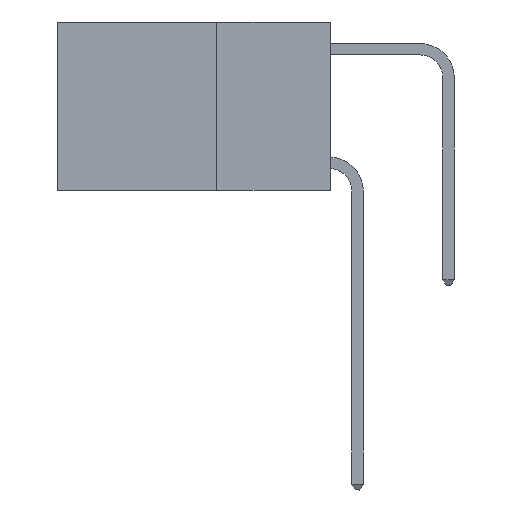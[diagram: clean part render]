
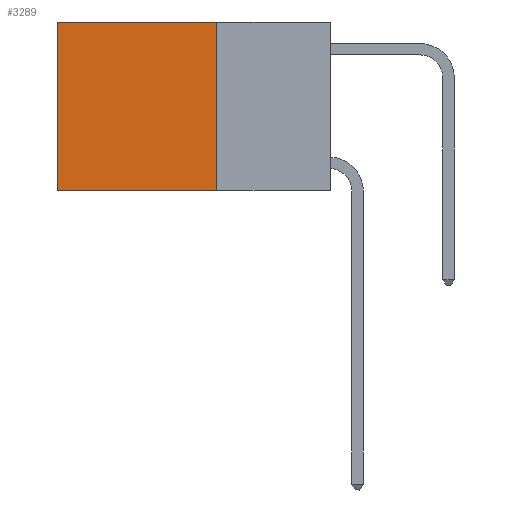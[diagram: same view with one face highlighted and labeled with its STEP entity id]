
A CAD part, left-side view. The second image highlights one B-rep face of the part: STEP entity #3289.
In plain terms, the highlighted planar face has unit normal (-1, 0, 0).
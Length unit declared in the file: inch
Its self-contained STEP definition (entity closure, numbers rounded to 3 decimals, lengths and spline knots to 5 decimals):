
#156 = PLANE ( 'NONE',  #4739 ) ;
#250 = LINE ( 'NONE', #12673, #16236 ) ;
#1476 = EDGE_LOOP ( 'NONE', ( #14057, #16489, #4400, #17234 ) ) ;
#1740 = DIRECTION ( 'NONE',  ( 0., 0., -1. ) ) ;
#2521 = VERTEX_POINT ( 'NONE', #5800 ) ;
#3289 = ADVANCED_FACE ( 'NONE', ( #7120 ), #156, .F. ) ;
#4400 = ORIENTED_EDGE ( 'NONE', *, *, #5109, .F. ) ;
#4739 = AXIS2_PLACEMENT_3D ( 'NONE', #4765, #10937, #1740 ) ;
#4765 = CARTESIAN_POINT ( 'NONE',  ( 0.2625, 0.25, 0. ) ) ;
#4880 = VECTOR ( 'NONE', #14399, 39.37008 ) ;
#5109 = EDGE_CURVE ( 'NONE', #18228, #11532, #250, .T. ) ;
#5800 = CARTESIAN_POINT ( 'NONE',  ( 0.2625, 0.6, 0. ) ) ;
#7120 = FACE_OUTER_BOUND ( 'NONE', #1476, .T. ) ;
#8067 = VECTOR ( 'NONE', #8450, 39.37008 ) ;
#8450 = DIRECTION ( 'NONE',  ( 0., 0., -1. ) ) ;
#8711 = EDGE_CURVE ( 'NONE', #18228, #2521, #14428, .T. ) ;
#9574 = CARTESIAN_POINT ( 'NONE',  ( 0.2625, 0.25, -0.37 ) ) ;
#10260 = VECTOR ( 'NONE', #14422, 39.37008 ) ;
#10937 = DIRECTION ( 'NONE',  ( 1., 0., 0. ) ) ;
#11504 = VERTEX_POINT ( 'NONE', #14237 ) ;
#11532 = VERTEX_POINT ( 'NONE', #9574 ) ;
#12673 = CARTESIAN_POINT ( 'NONE',  ( 0.2625, 0.25, 0. ) ) ;
#12789 = CARTESIAN_POINT ( 'NONE',  ( 0.2625, 0.25, -0.37 ) ) ;
#14057 = ORIENTED_EDGE ( 'NONE', *, *, #14212, .T. ) ;
#14212 = EDGE_CURVE ( 'NONE', #2521, #11504, #16334, .T. ) ;
#14237 = CARTESIAN_POINT ( 'NONE',  ( 0.2625, 0.6, -0.37 ) ) ;
#14399 = DIRECTION ( 'NONE',  ( 0., 1., 0. ) ) ;
#14418 = CARTESIAN_POINT ( 'NONE',  ( 0.2625, 0.25, 0. ) ) ;
#14422 = DIRECTION ( 'NONE',  ( 0., 1., 0. ) ) ;
#14428 = LINE ( 'NONE', #17497, #10260 ) ;
#16236 = VECTOR ( 'NONE', #17414, 39.37008 ) ;
#16334 = LINE ( 'NONE', #19218, #8067 ) ;
#16489 = ORIENTED_EDGE ( 'NONE', *, *, #19008, .F. ) ;
#16759 = LINE ( 'NONE', #12789, #4880 ) ;
#17234 = ORIENTED_EDGE ( 'NONE', *, *, #8711, .T. ) ;
#17414 = DIRECTION ( 'NONE',  ( 0., 0., -1. ) ) ;
#17497 = CARTESIAN_POINT ( 'NONE',  ( 0.2625, 0.25, 0. ) ) ;
#18228 = VERTEX_POINT ( 'NONE', #14418 ) ;
#19008 = EDGE_CURVE ( 'NONE', #11532, #11504, #16759, .T. ) ;
#19218 = CARTESIAN_POINT ( 'NONE',  ( 0.2625, 0.6, 0. ) ) ;
